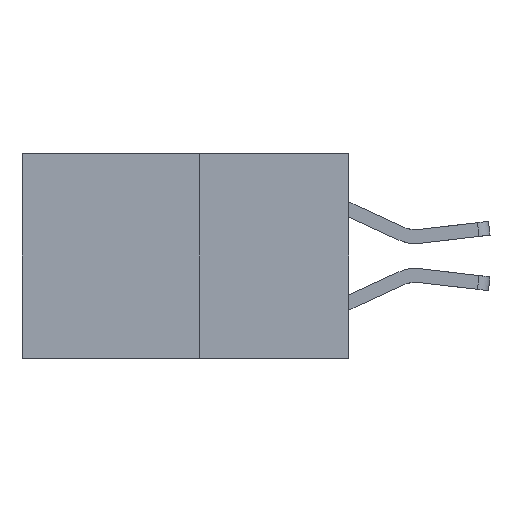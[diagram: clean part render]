
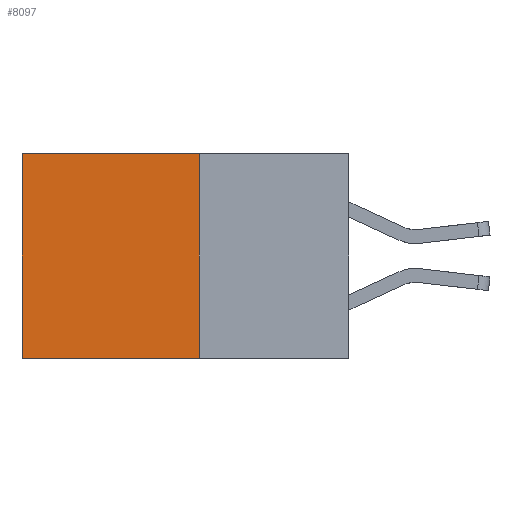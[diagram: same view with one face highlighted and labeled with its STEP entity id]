
A CAD part, left-side view. The second image highlights one B-rep face of the part: STEP entity #8097.
In plain terms, the highlighted planar face has unit normal (-1, 0, 0).
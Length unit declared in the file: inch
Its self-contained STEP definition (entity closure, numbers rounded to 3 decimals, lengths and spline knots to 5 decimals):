
#1184 = PLANE ( 'NONE',  #9856 ) ;
#1610 = EDGE_LOOP ( 'NONE', ( #10454, #13078, #10763, #13385 ) ) ;
#2206 = LINE ( 'NONE', #9975, #10222 ) ;
#2310 = DIRECTION ( 'NONE',  ( 0., 0., -1. ) ) ;
#3019 = DIRECTION ( 'NONE',  ( 0., 0., -1. ) ) ;
#3033 = VERTEX_POINT ( 'NONE', #13412 ) ;
#3474 = EDGE_CURVE ( 'NONE', #13083, #6951, #2206, .T. ) ;
#3780 = VERTEX_POINT ( 'NONE', #7397 ) ;
#4072 = CARTESIAN_POINT ( 'NONE',  ( 0.277, 0.27, -0.37 ) ) ;
#4223 = DIRECTION ( 'NONE',  ( 0., 0., -1. ) ) ;
#4466 = VECTOR ( 'NONE', #3019, 39.37008 ) ;
#5270 = CARTESIAN_POINT ( 'NONE',  ( 0.277, 0.59, -0.37 ) ) ;
#5741 = EDGE_CURVE ( 'NONE', #6951, #3780, #6455, .T. ) ;
#6382 = CARTESIAN_POINT ( 'NONE',  ( 0.277, 0.27, -0.37 ) ) ;
#6391 = EDGE_CURVE ( 'NONE', #13083, #3033, #12641, .T. ) ;
#6455 = LINE ( 'NONE', #5270, #11575 ) ;
#6951 = VERTEX_POINT ( 'NONE', #7951 ) ;
#7319 = EDGE_CURVE ( 'NONE', #3033, #3780, #9524, .T. ) ;
#7397 = CARTESIAN_POINT ( 'NONE',  ( 0.277, 0.59, -0.37 ) ) ;
#7580 = CARTESIAN_POINT ( 'NONE',  ( 0.277, 0.27, -0.37 ) ) ;
#7951 = CARTESIAN_POINT ( 'NONE',  ( 0.277, 0.59, 0. ) ) ;
#8097 = ADVANCED_FACE ( 'NONE', ( #12916 ), #1184, .F. ) ;
#8620 = DIRECTION ( 'NONE',  ( 1., 0., 0. ) ) ;
#8893 = VECTOR ( 'NONE', #11528, 39.37008 ) ;
#9524 = LINE ( 'NONE', #6382, #8893 ) ;
#9856 = AXIS2_PLACEMENT_3D ( 'NONE', #7580, #8620, #2310 ) ;
#9975 = CARTESIAN_POINT ( 'NONE',  ( 0.277, 0.27, 0. ) ) ;
#10000 = DIRECTION ( 'NONE',  ( 0., 1., 0. ) ) ;
#10222 = VECTOR ( 'NONE', #10000, 39.37008 ) ;
#10454 = ORIENTED_EDGE ( 'NONE', *, *, #5741, .T. ) ;
#10763 = ORIENTED_EDGE ( 'NONE', *, *, #6391, .F. ) ;
#11528 = DIRECTION ( 'NONE',  ( 0., 1., 0. ) ) ;
#11575 = VECTOR ( 'NONE', #4223, 39.37008 ) ;
#12266 = CARTESIAN_POINT ( 'NONE',  ( 0.277, 0.27, 0. ) ) ;
#12641 = LINE ( 'NONE', #4072, #4466 ) ;
#12916 = FACE_OUTER_BOUND ( 'NONE', #1610, .T. ) ;
#13078 = ORIENTED_EDGE ( 'NONE', *, *, #7319, .F. ) ;
#13083 = VERTEX_POINT ( 'NONE', #12266 ) ;
#13385 = ORIENTED_EDGE ( 'NONE', *, *, #3474, .T. ) ;
#13412 = CARTESIAN_POINT ( 'NONE',  ( 0.277, 0.27, -0.37 ) ) ;
